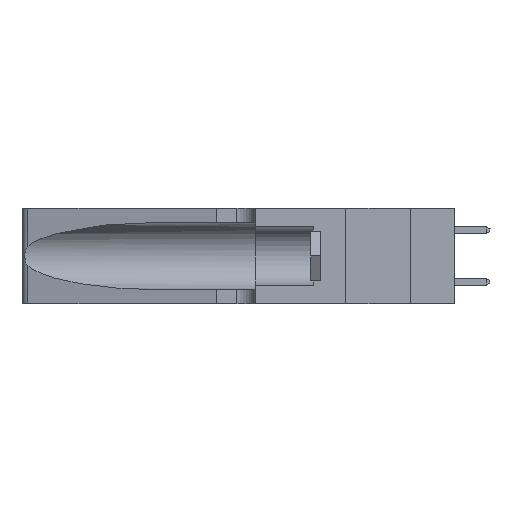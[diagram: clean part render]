
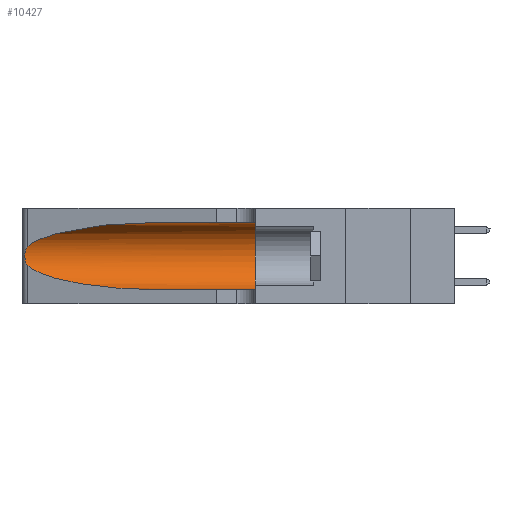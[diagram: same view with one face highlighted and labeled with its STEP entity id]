
A CAD part, left-side view. The second image highlights one B-rep face of the part: STEP entity #10427.
In plain terms, the highlighted cylindrical face has radius 3.308 mm (diameter 6.617 mm), a partial arc.
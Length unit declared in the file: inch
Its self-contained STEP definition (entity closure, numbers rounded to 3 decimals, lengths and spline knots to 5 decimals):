
#216 = AXIS2_PLACEMENT_3D ( 'NONE', #38772, #2811, #12914 ) ;
#311 = CARTESIAN_POINT ( 'NONE',  ( 0.1305, 0.72297, 0.31525 ) ) ;
#431 = ORIENTED_EDGE ( 'NONE', *, *, #8712, .T. ) ;
#521 = CARTESIAN_POINT ( 'NONE',  ( 0.26017, 1.23833, 0.17102 ) ) ;
#686 = CARTESIAN_POINT ( 'NONE',  ( 0.25856, 1.23593, 0.16098 ) ) ;
#840 = CARTESIAN_POINT ( 'NONE',  ( 0.25787, 1.23484, 0.2124 ) ) ;
#993 = CARTESIAN_POINT ( 'NONE',  ( 0.25639, 1.23184, 0.21858 ) ) ;
#2626 = CARTESIAN_POINT ( 'NONE',  ( 0.1305, 0.35, 0.05475 ) ) ;
#2670 = CARTESIAN_POINT ( 'NONE',  ( 0.25487, 1.22718, 0.14631 ) ) ;
#2811 = DIRECTION ( 'NONE',  ( 0., -1., 0. ) ) ;
#3144 = VERTEX_POINT ( 'NONE', #5014 ) ;
#4153 = ORIENTED_EDGE ( 'NONE', *, *, #12616, .F. ) ;
#4507 = CARTESIAN_POINT ( 'NONE',  ( 0.25555, 1.22993, 0.14849 ) ) ;
#4658 = CARTESIAN_POINT ( 'NONE',  ( 0.25487, 1.22718, 0.22369 ) ) ;
#4806 =( BOUNDED_CURVE ( )  B_SPLINE_CURVE ( 3, ( #21250, #42369, #9862, #20772 ),
 .UNSPECIFIED., .F., .F. ) 
 B_SPLINE_CURVE_WITH_KNOTS ( ( 4, 4 ),
 ( 3.44316, 4.71239 ),
 .UNSPECIFIED. ) 
 CURVE ( )  GEOMETRIC_REPRESENTATION_ITEM ( )  RATIONAL_B_SPLINE_CURVE ( ( 1., 0.87, 0.87, 1. ) ) 
 REPRESENTATION_ITEM ( '' )  );
#4885 = LINE ( 'NONE', #28513, #41148 ) ;
#5014 = CARTESIAN_POINT ( 'NONE',  ( 0.1305, 0.72297, 0.05475 ) ) ;
#5213 = LINE ( 'NONE', #8182, #25599 ) ;
#6801 = CIRCLE ( 'NONE', #35436, 0.13025 ) ;
#7194 = DIRECTION ( 'NONE',  ( 0., 1., 0. ) ) ;
#7818 = CARTESIAN_POINT ( 'NONE',  ( 0.26075, 1.23896, 0.178 ) ) ;
#8140 = CARTESIAN_POINT ( 'NONE',  ( 0.26075, 1.23896, 0.19203 ) ) ;
#8182 = CARTESIAN_POINT ( 'NONE',  ( 0.1305, 1.61858, 0.31525 ) ) ;
#8712 = EDGE_CURVE ( 'NONE', #28284, #43280, #13179, .T. ) ;
#9862 = CARTESIAN_POINT ( 'NONE',  ( 0.18966, 0.96281, 0.05475 ) ) ;
#10383 = CARTESIAN_POINT ( 'NONE',  ( 0.2373, 1.15595, 0.28018 ) ) ;
#10427 = ADVANCED_FACE ( 'NONE', ( #28184 ), #26516, .F. ) ;
#10851 = CARTESIAN_POINT ( 'NONE',  ( 0.1305, 0.35, 0.31525 ) ) ;
#11038 = VERTEX_POINT ( 'NONE', #2626 ) ;
#11246 = DIRECTION ( 'NONE',  ( 0., -1., 0. ) ) ;
#11436 = CARTESIAN_POINT ( 'NONE',  ( 0.26018, 1.23835, 0.19895 ) ) ;
#11848 = ORIENTED_EDGE ( 'NONE', *, *, #44254, .F. ) ;
#12616 = EDGE_CURVE ( 'NONE', #25786, #11038, #6801, .T. ) ;
#12914 = DIRECTION ( 'NONE',  ( 0., 0., -1. ) ) ;
#13179 = B_SPLINE_CURVE_WITH_KNOTS ( 'NONE', 3,
 ( #4658, #25867, #993, #840, #15383, #11436, #8140, #7818, #521, #686, #26476, #33138, #4507, #15076 ),
 .UNSPECIFIED., .F., .F.,
 ( 4, 2, 2, 2, 2, 2, 4 ),
 ( 0., 0.00027, 0.00053, 0.00107, 0.0016, 0.00187, 0.00214 ),
 .UNSPECIFIED. ) ;
#13387 = VERTEX_POINT ( 'NONE', #311 ) ;
#13611 = ORIENTED_EDGE ( 'NONE', *, *, #19017, .T. ) ;
#14329 = CARTESIAN_POINT ( 'NONE',  ( 0.25487, 1.22718, 0.22369 ) ) ;
#15076 = CARTESIAN_POINT ( 'NONE',  ( 0.25487, 1.22718, 0.14631 ) ) ;
#15383 = CARTESIAN_POINT ( 'NONE',  ( 0.25854, 1.2359, 0.20912 ) ) ;
#15582 = EDGE_CURVE ( 'NONE', #3144, #11038, #4885, .T. ) ;
#18708 = DIRECTION ( 'NONE',  ( 0., 0., 1. ) ) ;
#19017 = EDGE_CURVE ( 'NONE', #43280, #3144, #4806, .T. ) ;
#20772 = CARTESIAN_POINT ( 'NONE',  ( 0.1305, 0.72297, 0.05475 ) ) ;
#21250 = CARTESIAN_POINT ( 'NONE',  ( 0.25487, 1.22718, 0.14631 ) ) ;
#25599 = VECTOR ( 'NONE', #37008, 39.37008 ) ;
#25786 = VERTEX_POINT ( 'NONE', #10851 ) ;
#25867 = CARTESIAN_POINT ( 'NONE',  ( 0.25555, 1.22994, 0.2215 ) ) ;
#26476 = CARTESIAN_POINT ( 'NONE',  ( 0.25789, 1.23486, 0.15765 ) ) ;
#26516 = CYLINDRICAL_SURFACE ( 'NONE', #216, 0.13025 ) ;
#27531 = EDGE_CURVE ( 'NONE', #13387, #28284, #42857, .T. ) ;
#28184 = FACE_OUTER_BOUND ( 'NONE', #46359, .T. ) ;
#28284 = VERTEX_POINT ( 'NONE', #30268 ) ;
#28513 = CARTESIAN_POINT ( 'NONE',  ( 0.1305, 1.61858, 0.05475 ) ) ;
#30268 = CARTESIAN_POINT ( 'NONE',  ( 0.25487, 1.22718, 0.22369 ) ) ;
#32563 = CARTESIAN_POINT ( 'NONE',  ( 0.18966, 0.96281, 0.31525 ) ) ;
#33138 = CARTESIAN_POINT ( 'NONE',  ( 0.25639, 1.23186, 0.15144 ) ) ;
#33496 = ORIENTED_EDGE ( 'NONE', *, *, #27531, .T. ) ;
#35436 = AXIS2_PLACEMENT_3D ( 'NONE', #39818, #7194, #18708 ) ;
#37008 = DIRECTION ( 'NONE',  ( 0., -1., 0. ) ) ;
#38772 = CARTESIAN_POINT ( 'NONE',  ( 0.1305, 1.61858, 0.185 ) ) ;
#39818 = CARTESIAN_POINT ( 'NONE',  ( 0.1305, 0.35, 0.185 ) ) ;
#41148 = VECTOR ( 'NONE', #11246, 39.37008 ) ;
#42369 = CARTESIAN_POINT ( 'NONE',  ( 0.2373, 1.15595, 0.08982 ) ) ;
#42857 =( BOUNDED_CURVE ( )  B_SPLINE_CURVE ( 3, ( #43235, #32563, #10383, #14329 ),
 .UNSPECIFIED., .F., .F. ) 
 B_SPLINE_CURVE_WITH_KNOTS ( ( 4, 4 ),
 ( 1.5708, 2.84003 ),
 .UNSPECIFIED. ) 
 CURVE ( )  GEOMETRIC_REPRESENTATION_ITEM ( )  RATIONAL_B_SPLINE_CURVE ( ( 1., 0.87, 0.87, 1. ) ) 
 REPRESENTATION_ITEM ( '' )  );
#43235 = CARTESIAN_POINT ( 'NONE',  ( 0.1305, 0.72297, 0.31525 ) ) ;
#43280 = VERTEX_POINT ( 'NONE', #2670 ) ;
#44254 = EDGE_CURVE ( 'NONE', #13387, #25786, #5213, .T. ) ;
#46359 = EDGE_LOOP ( 'NONE', ( #33496, #431, #13611, #46586, #4153, #11848 ) ) ;
#46586 = ORIENTED_EDGE ( 'NONE', *, *, #15582, .T. ) ;
